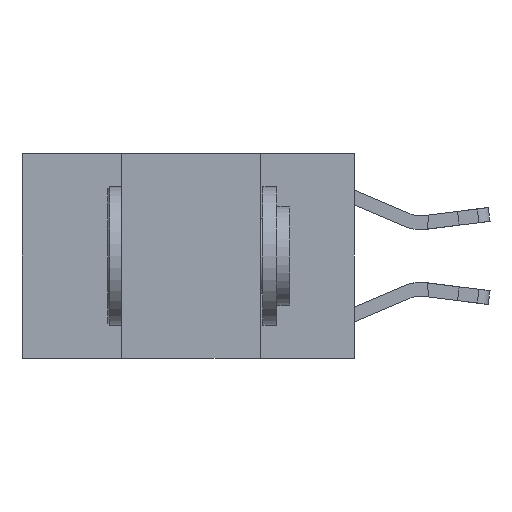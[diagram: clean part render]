
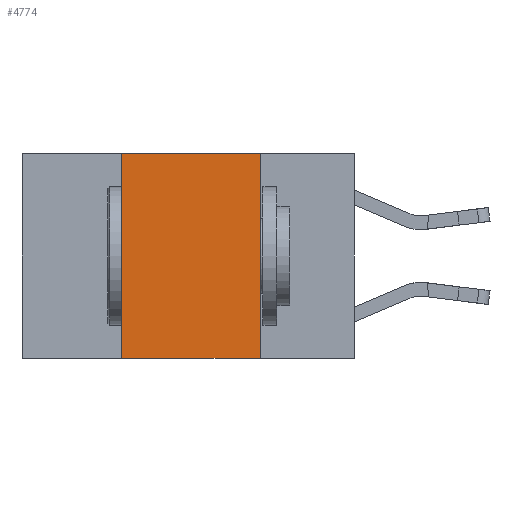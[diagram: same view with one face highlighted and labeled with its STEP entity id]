
A CAD part, left-side view. The second image highlights one B-rep face of the part: STEP entity #4774.
In plain terms, the highlighted planar face has unit normal (-1, 0, 0).
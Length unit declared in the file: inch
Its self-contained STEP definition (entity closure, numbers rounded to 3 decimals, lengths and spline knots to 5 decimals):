
#794 = LINE ( 'NONE', #12983, #14680 ) ;
#934 = EDGE_CURVE ( 'NONE', #15989, #1684, #13121, .T. ) ;
#1684 = VERTEX_POINT ( 'NONE', #13749 ) ;
#1819 = DIRECTION ( 'NONE',  ( 0., -1., 0. ) ) ;
#2777 = VERTEX_POINT ( 'NONE', #11225 ) ;
#3045 = CARTESIAN_POINT ( 'NONE',  ( 0., 0.42, 0. ) ) ;
#3307 = LINE ( 'NONE', #5527, #3969 ) ;
#3525 = EDGE_CURVE ( 'NONE', #11591, #2777, #3307, .T. ) ;
#3718 = ORIENTED_EDGE ( 'NONE', *, *, #15394, .F. ) ;
#3969 = VECTOR ( 'NONE', #7958, 39.37008 ) ;
#4160 = CARTESIAN_POINT ( 'NONE',  ( 0., 0.6, 0. ) ) ;
#4275 = AXIS2_PLACEMENT_3D ( 'NONE', #4160, #11562, #9073 ) ;
#4774 = ADVANCED_FACE ( 'NONE', ( #12862 ), #14069, .F. ) ;
#5517 = CARTESIAN_POINT ( 'NONE',  ( 0., 0.17, 0. ) ) ;
#5527 = CARTESIAN_POINT ( 'NONE',  ( 0., 0.17, 0. ) ) ;
#5832 = CARTESIAN_POINT ( 'NONE',  ( 0., 0.42, -0.37 ) ) ;
#6372 = DIRECTION ( 'NONE',  ( 0., -1., 0. ) ) ;
#7594 = ORIENTED_EDGE ( 'NONE', *, *, #14796, .T. ) ;
#7958 = DIRECTION ( 'NONE',  ( 0., 0., -1. ) ) ;
#8106 = ORIENTED_EDGE ( 'NONE', *, *, #934, .F. ) ;
#8521 = ORIENTED_EDGE ( 'NONE', *, *, #3525, .F. ) ;
#9009 = VECTOR ( 'NONE', #6372, 39.37008 ) ;
#9073 = DIRECTION ( 'NONE',  ( 0., 0., -1. ) ) ;
#9405 = DIRECTION ( 'NONE',  ( 0., 0., 1. ) ) ;
#10429 = LINE ( 'NONE', #13979, #9009 ) ;
#10625 = EDGE_LOOP ( 'NONE', ( #8521, #3718, #8106, #7594 ) ) ;
#11174 = VECTOR ( 'NONE', #9405, 39.37008 ) ;
#11225 = CARTESIAN_POINT ( 'NONE',  ( 0., 0.17, -0.37 ) ) ;
#11562 = DIRECTION ( 'NONE',  ( 1., 0., 0. ) ) ;
#11591 = VERTEX_POINT ( 'NONE', #5517 ) ;
#12862 = FACE_OUTER_BOUND ( 'NONE', #10625, .T. ) ;
#12983 = CARTESIAN_POINT ( 'NONE',  ( 0., 0.6, 0. ) ) ;
#13121 = LINE ( 'NONE', #3045, #11174 ) ;
#13749 = CARTESIAN_POINT ( 'NONE',  ( 0., 0.42, 0. ) ) ;
#13979 = CARTESIAN_POINT ( 'NONE',  ( 0., 0.6, -0.37 ) ) ;
#14069 = PLANE ( 'NONE',  #4275 ) ;
#14680 = VECTOR ( 'NONE', #1819, 39.37008 ) ;
#14796 = EDGE_CURVE ( 'NONE', #15989, #2777, #10429, .T. ) ;
#15394 = EDGE_CURVE ( 'NONE', #1684, #11591, #794, .T. ) ;
#15989 = VERTEX_POINT ( 'NONE', #5832 ) ;
